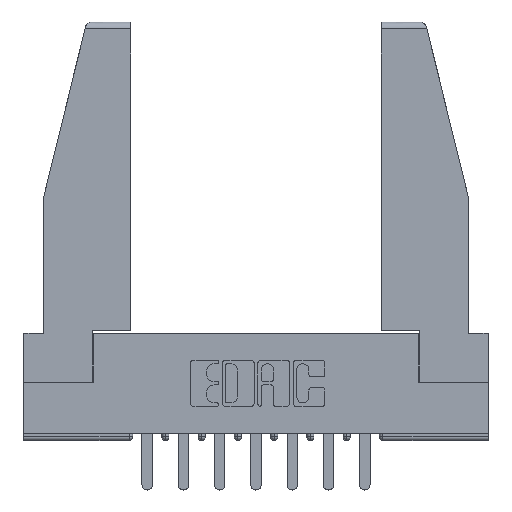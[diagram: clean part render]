
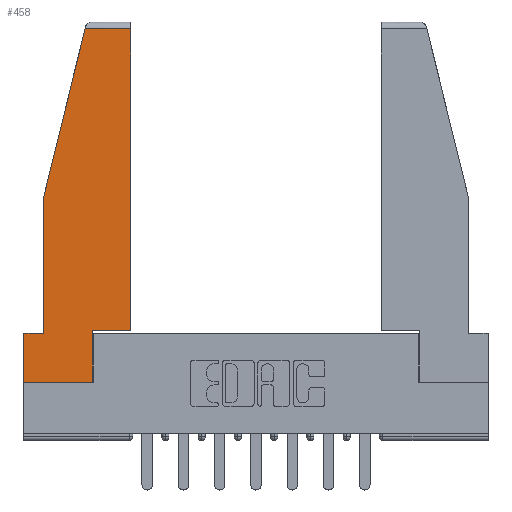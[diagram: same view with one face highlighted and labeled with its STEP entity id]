
A CAD part, top view. The second image highlights one B-rep face of the part: STEP entity #458.
In plain terms, the highlighted planar face has unit normal (0, 0, 1).
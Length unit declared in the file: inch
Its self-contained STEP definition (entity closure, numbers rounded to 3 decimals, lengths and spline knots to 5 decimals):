
#52 = ORIENTED_EDGE ( 'NONE', *, *, #1675, .T. ) ;
#288 = EDGE_CURVE ( 'NONE', #1924, #399, #869, .T. ) ;
#399 = VERTEX_POINT ( 'NONE', #657 ) ;
#458 = ADVANCED_FACE ( 'NONE', ( #4816 ), #1551, .T. ) ;
#510 = ORIENTED_EDGE ( 'NONE', *, *, #288, .T. ) ;
#657 = CARTESIAN_POINT ( 'NONE',  ( 0., 0., 0. ) ) ;
#672 = EDGE_CURVE ( 'NONE', #1065, #12495, #6353, .T. ) ;
#690 = ORIENTED_EDGE ( 'NONE', *, *, #13752, .T. ) ;
#821 = VERTEX_POINT ( 'NONE', #11005 ) ;
#869 = LINE ( 'NONE', #1415, #2570 ) ;
#1065 = VERTEX_POINT ( 'NONE', #10372 ) ;
#1170 = DIRECTION ( 'NONE',  ( 1., 0., 0. ) ) ;
#1415 = CARTESIAN_POINT ( 'NONE',  ( 0., 0.21, 0. ) ) ;
#1551 = PLANE ( 'NONE',  #13693 ) ;
#1675 = EDGE_CURVE ( 'NONE', #12495, #1924, #10467, .T. ) ;
#1910 = CARTESIAN_POINT ( 'NONE',  ( 0.297, 0., 0. ) ) ;
#1924 = VERTEX_POINT ( 'NONE', #7276 ) ;
#2405 = ORIENTED_EDGE ( 'NONE', *, *, #672, .T. ) ;
#2425 = ORIENTED_EDGE ( 'NONE', *, *, #14031, .T. ) ;
#2526 = VECTOR ( 'NONE', #5963, 39.37008 ) ;
#2570 = VECTOR ( 'NONE', #10204, 39.37008 ) ;
#2641 = DIRECTION ( 'NONE',  ( 0., 0., 1. ) ) ;
#3129 = EDGE_LOOP ( 'NONE', ( #4943, #690, #4698, #2405, #52, #510, #3610, #6391, #2425 ) ) ;
#3133 = CARTESIAN_POINT ( 'NONE',  ( 0.461, 0.223, 0. ) ) ;
#3157 = CARTESIAN_POINT ( 'NONE',  ( 0.461, 1.52, 0. ) ) ;
#3455 = VECTOR ( 'NONE', #14086, 39.37008 ) ;
#3610 = ORIENTED_EDGE ( 'NONE', *, *, #5912, .T. ) ;
#3877 = EDGE_CURVE ( 'NONE', #821, #1065, #9023, .T. ) ;
#4019 = CARTESIAN_POINT ( 'NONE',  ( 0., 0., 0. ) ) ;
#4195 = CARTESIAN_POINT ( 'NONE',  ( 0.086, 0.21, 0. ) ) ;
#4262 = DIRECTION ( 'NONE',  ( 1., 0., 0. ) ) ;
#4569 = CARTESIAN_POINT ( 'NONE',  ( 0., 0.21, 0. ) ) ;
#4698 = ORIENTED_EDGE ( 'NONE', *, *, #3877, .T. ) ;
#4754 = DIRECTION ( 'NONE',  ( 0., 1., 0. ) ) ;
#4816 = FACE_OUTER_BOUND ( 'NONE', #3129, .T. ) ;
#4832 = CARTESIAN_POINT ( 'NONE',  ( 0.297, 0., 0. ) ) ;
#4923 = LINE ( 'NONE', #4832, #2526 ) ;
#4943 = ORIENTED_EDGE ( 'NONE', *, *, #6399, .T. ) ;
#5066 = VECTOR ( 'NONE', #11268, 39.37008 ) ;
#5138 = LINE ( 'NONE', #10050, #13021 ) ;
#5474 = CARTESIAN_POINT ( 'NONE',  ( 0.086, 0.8, 0. ) ) ;
#5912 = EDGE_CURVE ( 'NONE', #399, #9714, #10340, .T. ) ;
#5914 = DIRECTION ( 'NONE',  ( -1., 0., 0. ) ) ;
#5963 = DIRECTION ( 'NONE',  ( 0., 1., 0. ) ) ;
#6353 = LINE ( 'NONE', #5474, #3455 ) ;
#6391 = ORIENTED_EDGE ( 'NONE', *, *, #9825, .T. ) ;
#6399 = EDGE_CURVE ( 'NONE', #10092, #12866, #10638, .T. ) ;
#6850 = VECTOR ( 'NONE', #5914, 39.37008 ) ;
#6876 = CARTESIAN_POINT ( 'NONE',  ( 0.271, 1.55, 0. ) ) ;
#7003 = CARTESIAN_POINT ( 'NONE',  ( 0., 0., 0. ) ) ;
#7018 = LINE ( 'NONE', #8088, #6850 ) ;
#7097 = DIRECTION ( 'NONE',  ( 1., 0., 0. ) ) ;
#7276 = CARTESIAN_POINT ( 'NONE',  ( 0., 0.21, 0. ) ) ;
#7849 = CARTESIAN_POINT ( 'NONE',  ( 0.297, 0.223, 0. ) ) ;
#8088 = CARTESIAN_POINT ( 'NONE',  ( 0., 1.52, 0. ) ) ;
#8213 = DIRECTION ( 'NONE',  ( -1., 0., 0. ) ) ;
#8600 = VECTOR ( 'NONE', #4262, 39.37008 ) ;
#9023 = LINE ( 'NONE', #6876, #5066 ) ;
#9714 = VERTEX_POINT ( 'NONE', #1910 ) ;
#9772 = VECTOR ( 'NONE', #8213, 39.37008 ) ;
#9825 = EDGE_CURVE ( 'NONE', #9714, #11543, #4923, .T. ) ;
#10050 = CARTESIAN_POINT ( 'NONE',  ( 0.297, 0.223, 0. ) ) ;
#10092 = VERTEX_POINT ( 'NONE', #3133 ) ;
#10204 = DIRECTION ( 'NONE',  ( 0., -1., 0. ) ) ;
#10340 = LINE ( 'NONE', #4019, #8600 ) ;
#10372 = CARTESIAN_POINT ( 'NONE',  ( 0.086, 0.8, 0. ) ) ;
#10467 = LINE ( 'NONE', #4569, #9772 ) ;
#10638 = LINE ( 'NONE', #12376, #13199 ) ;
#11005 = CARTESIAN_POINT ( 'NONE',  ( 0.2636, 1.52, 0. ) ) ;
#11268 = DIRECTION ( 'NONE',  ( -0.239, -0.971, 0. ) ) ;
#11543 = VERTEX_POINT ( 'NONE', #7849 ) ;
#12376 = CARTESIAN_POINT ( 'NONE',  ( 0.461, 0.223, 0. ) ) ;
#12495 = VERTEX_POINT ( 'NONE', #4195 ) ;
#12866 = VERTEX_POINT ( 'NONE', #3157 ) ;
#13021 = VECTOR ( 'NONE', #1170, 39.37008 ) ;
#13199 = VECTOR ( 'NONE', #4754, 39.37008 ) ;
#13693 = AXIS2_PLACEMENT_3D ( 'NONE', #7003, #2641, #7097 ) ;
#13752 = EDGE_CURVE ( 'NONE', #12866, #821, #7018, .T. ) ;
#14031 = EDGE_CURVE ( 'NONE', #11543, #10092, #5138, .T. ) ;
#14086 = DIRECTION ( 'NONE',  ( 0., -1., 0. ) ) ;
